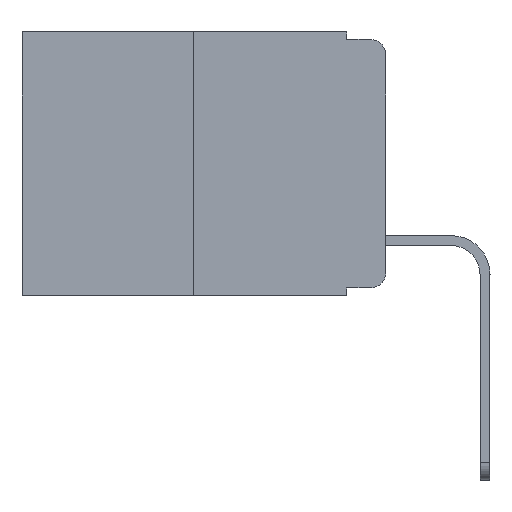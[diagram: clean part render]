
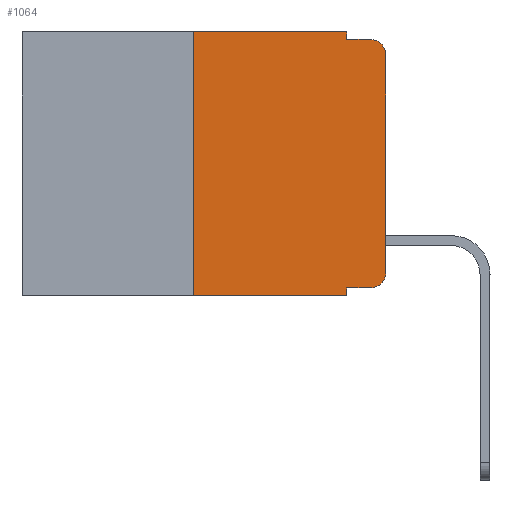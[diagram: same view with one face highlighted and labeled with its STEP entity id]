
A CAD part, left-side view. The second image highlights one B-rep face of the part: STEP entity #1064.
In plain terms, the highlighted planar face has unit normal (-1, 0, 0).
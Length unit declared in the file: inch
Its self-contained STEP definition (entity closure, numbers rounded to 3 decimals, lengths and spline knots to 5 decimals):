
#514 = VERTEX_POINT ( 'NONE', #4043 ) ;
#672 = CARTESIAN_POINT ( 'NONE',  ( 0., 0.25, -0.343 ) ) ;
#777 = DIRECTION ( 'NONE',  ( 0., 0., -1. ) ) ;
#996 = ORIENTED_EDGE ( 'NONE', *, *, #1794, .T. ) ;
#1064 = ADVANCED_FACE ( 'NONE', ( #1138 ), #13549, .F. ) ;
#1138 = FACE_OUTER_BOUND ( 'NONE', #4080, .T. ) ;
#1186 = LINE ( 'NONE', #2389, #12223 ) ;
#1476 = CARTESIAN_POINT ( 'NONE',  ( 0., 0.02, -0.03 ) ) ;
#1491 = EDGE_CURVE ( 'NONE', #11857, #5606, #2655, .T. ) ;
#1495 = LINE ( 'NONE', #11651, #12195 ) ;
#1561 = CARTESIAN_POINT ( 'NONE',  ( 0., 0.25, 0. ) ) ;
#1626 = VECTOR ( 'NONE', #2931, 39.37008 ) ;
#1794 = EDGE_CURVE ( 'NONE', #514, #8425, #5799, .T. ) ;
#1833 = CARTESIAN_POINT ( 'NONE',  ( 0., 0., -0.313 ) ) ;
#1843 = EDGE_CURVE ( 'NONE', #11496, #11105, #13471, .T. ) ;
#2011 = CARTESIAN_POINT ( 'NONE',  ( 0., 0.02, -0.313 ) ) ;
#2101 = CARTESIAN_POINT ( 'NONE',  ( 0., 0.02, -0.333 ) ) ;
#2231 = AXIS2_PLACEMENT_3D ( 'NONE', #6191, #5237, #777 ) ;
#2389 = CARTESIAN_POINT ( 'NONE',  ( 0., 0.051, 0. ) ) ;
#2454 = VERTEX_POINT ( 'NONE', #10424 ) ;
#2509 = CARTESIAN_POINT ( 'NONE',  ( 0., 0.473, -0.343 ) ) ;
#2625 = ORIENTED_EDGE ( 'NONE', *, *, #4808, .F. ) ;
#2638 = CARTESIAN_POINT ( 'NONE',  ( 0., 0.051, -0.333 ) ) ;
#2655 = LINE ( 'NONE', #9407, #1626 ) ;
#2687 = LINE ( 'NONE', #9050, #4849 ) ;
#2931 = DIRECTION ( 'NONE',  ( 0., 0., -1. ) ) ;
#2988 = CARTESIAN_POINT ( 'NONE',  ( 0., 0.051, -0.01 ) ) ;
#3943 = LINE ( 'NONE', #2509, #7474 ) ;
#4040 = VECTOR ( 'NONE', #4739, 39.37008 ) ;
#4043 = CARTESIAN_POINT ( 'NONE',  ( 0., 0.051, -0.333 ) ) ;
#4080 = EDGE_LOOP ( 'NONE', ( #5858, #9777, #7916, #4595, #10615, #5600, #12210, #2625, #996, #7355 ) ) ;
#4360 = CARTESIAN_POINT ( 'NONE',  ( 0., 0.25, 0. ) ) ;
#4595 = ORIENTED_EDGE ( 'NONE', *, *, #1491, .F. ) ;
#4739 = DIRECTION ( 'NONE',  ( 0., -1., 0. ) ) ;
#4808 = EDGE_CURVE ( 'NONE', #514, #6610, #1186, .T. ) ;
#4849 = VECTOR ( 'NONE', #6753, 39.37008 ) ;
#5043 = VERTEX_POINT ( 'NONE', #1833 ) ;
#5237 = DIRECTION ( 'NONE',  ( 1., 0., 0. ) ) ;
#5600 = ORIENTED_EDGE ( 'NONE', *, *, #1843, .F. ) ;
#5606 = VERTEX_POINT ( 'NONE', #2988 ) ;
#5799 = LINE ( 'NONE', #2638, #10976 ) ;
#5858 = ORIENTED_EDGE ( 'NONE', *, *, #8434, .T. ) ;
#6022 = EDGE_CURVE ( 'NONE', #5606, #6042, #2687, .T. ) ;
#6042 = VERTEX_POINT ( 'NONE', #9002 ) ;
#6069 = EDGE_CURVE ( 'NONE', #2454, #6042, #12855, .T. ) ;
#6123 = VECTOR ( 'NONE', #8058, 39.37008 ) ;
#6191 = CARTESIAN_POINT ( 'NONE',  ( 0., 0.473, 0. ) ) ;
#6610 = VERTEX_POINT ( 'NONE', #9034 ) ;
#6647 = DIRECTION ( 'NONE',  ( 0., 0., -1. ) ) ;
#6753 = DIRECTION ( 'NONE',  ( 0., -1., 0. ) ) ;
#7355 = ORIENTED_EDGE ( 'NONE', *, *, #12149, .T. ) ;
#7474 = VECTOR ( 'NONE', #11041, 39.37008 ) ;
#7570 = LINE ( 'NONE', #8996, #4040 ) ;
#7916 = ORIENTED_EDGE ( 'NONE', *, *, #6022, .F. ) ;
#8058 = DIRECTION ( 'NONE',  ( 0., 0., 1. ) ) ;
#8425 = VERTEX_POINT ( 'NONE', #2101 ) ;
#8434 = EDGE_CURVE ( 'NONE', #5043, #2454, #1495, .T. ) ;
#8949 = DIRECTION ( 'NONE',  ( -1., 0., 0. ) ) ;
#8996 = CARTESIAN_POINT ( 'NONE',  ( 0., 0.473, 0. ) ) ;
#9002 = CARTESIAN_POINT ( 'NONE',  ( 0., 0.02, -0.01 ) ) ;
#9034 = CARTESIAN_POINT ( 'NONE',  ( 0., 0.051, -0.343 ) ) ;
#9050 = CARTESIAN_POINT ( 'NONE',  ( 0., 0.051, -0.01 ) ) ;
#9407 = CARTESIAN_POINT ( 'NONE',  ( 0., 0.051, 0. ) ) ;
#9652 = AXIS2_PLACEMENT_3D ( 'NONE', #2011, #13673, #10582 ) ;
#9777 = ORIENTED_EDGE ( 'NONE', *, *, #6069, .T. ) ;
#9945 = EDGE_CURVE ( 'NONE', #11105, #11857, #7570, .T. ) ;
#10022 = DIRECTION ( 'NONE',  ( 0., -1., 0. ) ) ;
#10424 = CARTESIAN_POINT ( 'NONE',  ( 0., 0., -0.03 ) ) ;
#10582 = DIRECTION ( 'NONE',  ( 0., 0., -1. ) ) ;
#10615 = ORIENTED_EDGE ( 'NONE', *, *, #9945, .F. ) ;
#10976 = VECTOR ( 'NONE', #10022, 39.37008 ) ;
#11041 = DIRECTION ( 'NONE',  ( 0., -1., 0. ) ) ;
#11105 = VERTEX_POINT ( 'NONE', #4360 ) ;
#11496 = VERTEX_POINT ( 'NONE', #672 ) ;
#11651 = CARTESIAN_POINT ( 'NONE',  ( 0., 0., 0. ) ) ;
#11857 = VERTEX_POINT ( 'NONE', #12883 ) ;
#12149 = EDGE_CURVE ( 'NONE', #8425, #5043, #12160, .T. ) ;
#12160 = CIRCLE ( 'NONE', #9652, 0.02 ) ;
#12195 = VECTOR ( 'NONE', #13678, 39.37008 ) ;
#12210 = ORIENTED_EDGE ( 'NONE', *, *, #13741, .T. ) ;
#12223 = VECTOR ( 'NONE', #6647, 39.37008 ) ;
#12855 = CIRCLE ( 'NONE', #13081, 0.02 ) ;
#12883 = CARTESIAN_POINT ( 'NONE',  ( 0., 0.051, 0. ) ) ;
#13081 = AXIS2_PLACEMENT_3D ( 'NONE', #1476, #8949, #13082 ) ;
#13082 = DIRECTION ( 'NONE',  ( 0., 0., -1. ) ) ;
#13471 = LINE ( 'NONE', #1561, #6123 ) ;
#13549 = PLANE ( 'NONE',  #2231 ) ;
#13673 = DIRECTION ( 'NONE',  ( -1., 0., 0. ) ) ;
#13678 = DIRECTION ( 'NONE',  ( 0., 0., 1. ) ) ;
#13741 = EDGE_CURVE ( 'NONE', #11496, #6610, #3943, .T. ) ;
